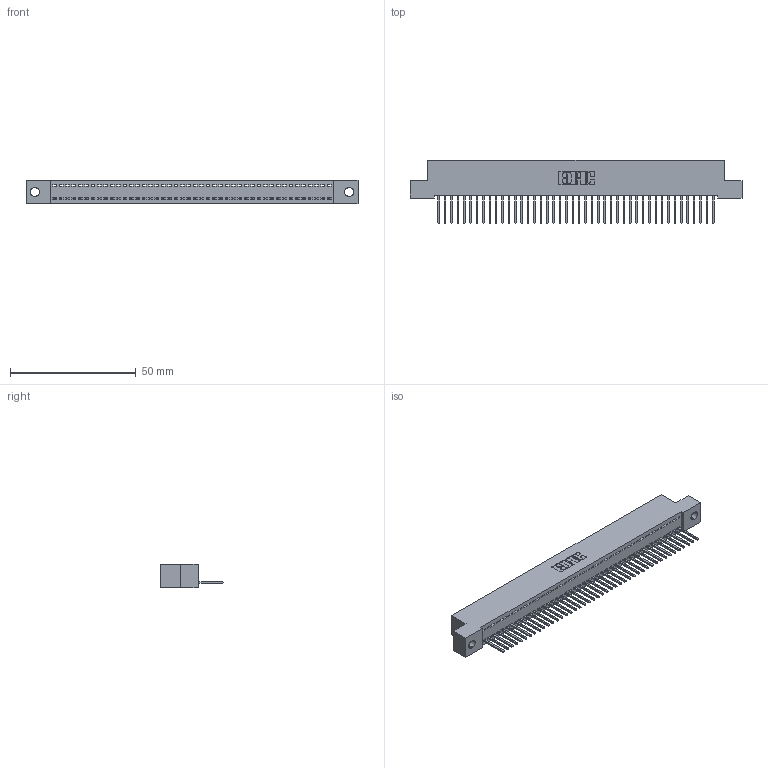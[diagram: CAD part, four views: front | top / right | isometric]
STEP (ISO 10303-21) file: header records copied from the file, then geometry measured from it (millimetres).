
FILE_DESCRIPTION (( 'STEP AP203' ), '1' );
FILE_NAME ('342-044-523-102.STEP', '2019-10-02T19:00:32', ( '' ), ( '' ), 'SwSTEP 2.0', 'SolidWorks 2016', '' );
FILE_SCHEMA (( 'CONFIG_CONTROL_DESIGN' ));
Length unit declared in the file: inch
Products named in the file (3): 342-044-523-102; 342 Part_.128 Slot; 345-292-001_345-293-123
Assembly tree (45 placements, depth 2):
  342-044-523-102
    342 Part_.128 Slot
    345-292-001_345-293-123  x44
Bounding box: 132.08 x 25.15 x 9.4 mm (x, y, z)
Volume: 11519 mm3; surface area: 16754 mm2
Topology: 45 solids, 45 shells, 2666 faces, 8055 edges, 5310 vertices
Faces by surface type: plane 1918, cylinder 748
Entity records: 26661 total; most frequent: CARTESIAN_POINT 4606, ORIENTED_EDGE 4586, DIRECTION 3881, EDGE_CURVE 2293, LINE 2165, VECTOR 2165, VERTEX_POINT 1526, AXIS2_PLACEMENT_3D 858
